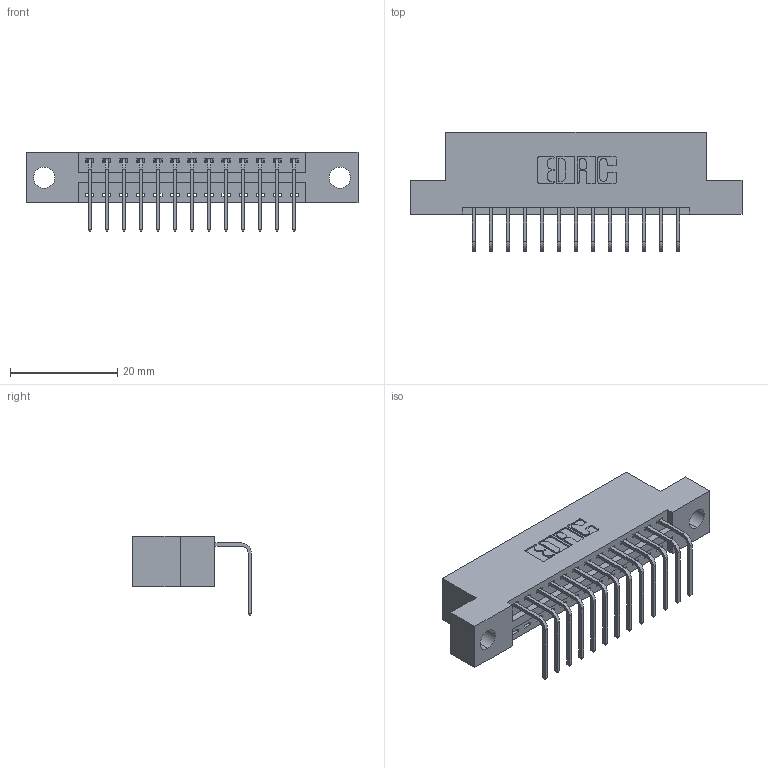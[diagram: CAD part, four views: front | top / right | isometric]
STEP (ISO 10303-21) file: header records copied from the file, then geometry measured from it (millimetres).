
FILE_DESCRIPTION (( 'STEP AP203' ), '1' );
FILE_NAME ('346-013-558-104.STEP', '2022-05-05T05:04:40', ( '' ), ( '' ), 'SwSTEP 2.0', 'SolidWorks 2020', '' );
FILE_SCHEMA (( 'CONFIG_CONTROL_DESIGN' ));
Length unit declared in the file: inch
Products named in the file (3): 345-292-001_558 Tail - 2; 346-013-558-104; 346 Part_Flush Mounting Lugs - 0.156 Dia-TH
Assembly tree (14 placements, depth 2):
  346-013-558-104
    346 Part_Flush Mounting Lugs - 0.156 Dia-TH
    345-292-001_558 Tail - 2  x13
Bounding box: 61.85 x 22.16 x 14.73 mm (x, y, z)
Volume: 5657.9 mm3; surface area: 6854.3 mm2
Topology: 14 solids, 14 shells, 916 faces, 2731 edges, 1802 vertices
Faces by surface type: plane 636, cylinder 280
Entity records: 12475 total; most frequent: CARTESIAN_POINT 2157, ORIENTED_EDGE 2102, DIRECTION 1937, EDGE_CURVE 1051, LINE 867, VECTOR 867, VERTEX_POINT 698, AXIS2_PLACEMENT_3D 535
